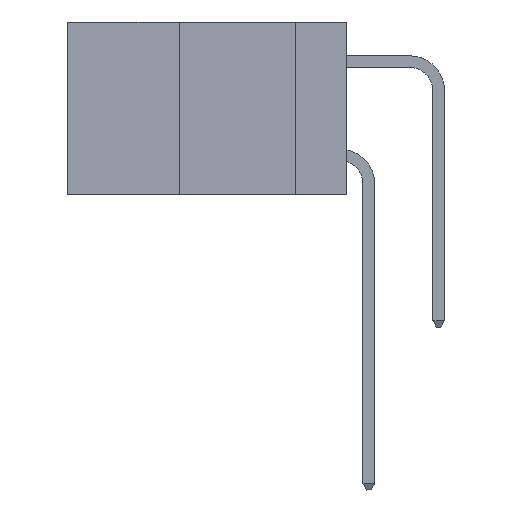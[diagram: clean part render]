
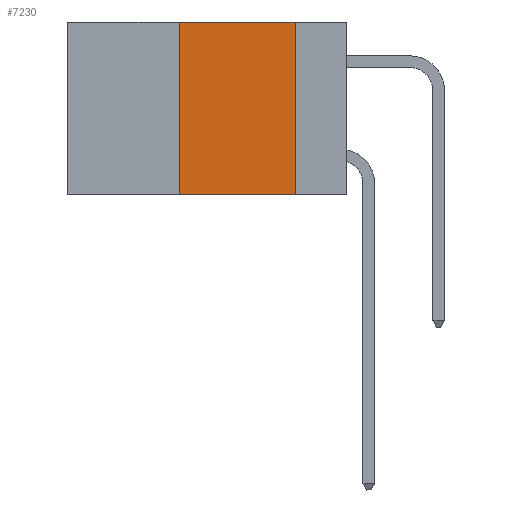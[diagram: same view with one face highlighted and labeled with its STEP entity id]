
A CAD part, left-side view. The second image highlights one B-rep face of the part: STEP entity #7230.
In plain terms, the highlighted planar face has unit normal (-1, 0, 0).
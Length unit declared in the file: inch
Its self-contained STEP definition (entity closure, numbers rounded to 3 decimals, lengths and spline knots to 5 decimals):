
#558 = VERTEX_POINT ( 'NONE', #15629 ) ;
#1822 = ORIENTED_EDGE ( 'NONE', *, *, #13832, .T. ) ;
#1832 = DIRECTION ( 'NONE',  ( 0., 0., -1. ) ) ;
#1865 = FACE_OUTER_BOUND ( 'NONE', #11019, .T. ) ;
#2364 = CARTESIAN_POINT ( 'NONE',  ( 0., 0.6, -0.37 ) ) ;
#2474 = DIRECTION ( 'NONE',  ( 0., -1., 0. ) ) ;
#3385 = VERTEX_POINT ( 'NONE', #8824 ) ;
#3894 = DIRECTION ( 'NONE',  ( 0., -1., 0. ) ) ;
#4068 = CARTESIAN_POINT ( 'NONE',  ( 0., 0.6, 0. ) ) ;
#4697 = VECTOR ( 'NONE', #3894, 39.37008 ) ;
#5134 = ORIENTED_EDGE ( 'NONE', *, *, #15643, .F. ) ;
#5179 = LINE ( 'NONE', #2364, #4697 ) ;
#6358 = CARTESIAN_POINT ( 'NONE',  ( 0., 0.11, 0. ) ) ;
#6613 = VERTEX_POINT ( 'NONE', #8448 ) ;
#6871 = VERTEX_POINT ( 'NONE', #9005 ) ;
#6977 = EDGE_CURVE ( 'NONE', #6871, #558, #10029, .T. ) ;
#6983 = PLANE ( 'NONE',  #18477 ) ;
#7230 = ADVANCED_FACE ( 'NONE', ( #1865 ), #6983, .F. ) ;
#7752 = VECTOR ( 'NONE', #2474, 39.37008 ) ;
#8200 = LINE ( 'NONE', #4068, #7752 ) ;
#8424 = DIRECTION ( 'NONE',  ( 0., 0., -1. ) ) ;
#8448 = CARTESIAN_POINT ( 'NONE',  ( 0., 0.36, -0.37 ) ) ;
#8824 = CARTESIAN_POINT ( 'NONE',  ( 0., 0.36, 0. ) ) ;
#9005 = CARTESIAN_POINT ( 'NONE',  ( 0., 0.11, 0. ) ) ;
#9834 = CARTESIAN_POINT ( 'NONE',  ( 0., 0.6, 0. ) ) ;
#10022 = CARTESIAN_POINT ( 'NONE',  ( 0., 0.36, 0. ) ) ;
#10029 = LINE ( 'NONE', #6358, #17221 ) ;
#11019 = EDGE_LOOP ( 'NONE', ( #17334, #18009, #5134, #1822 ) ) ;
#12749 = EDGE_CURVE ( 'NONE', #3385, #6871, #8200, .T. ) ;
#13832 = EDGE_CURVE ( 'NONE', #6613, #558, #5179, .T. ) ;
#13918 = VECTOR ( 'NONE', #16676, 39.37008 ) ;
#14335 = LINE ( 'NONE', #10022, #13918 ) ;
#15629 = CARTESIAN_POINT ( 'NONE',  ( 0., 0.11, -0.37 ) ) ;
#15643 = EDGE_CURVE ( 'NONE', #6613, #3385, #14335, .T. ) ;
#16617 = DIRECTION ( 'NONE',  ( 1., 0., 0. ) ) ;
#16676 = DIRECTION ( 'NONE',  ( 0., 0., 1. ) ) ;
#17221 = VECTOR ( 'NONE', #1832, 39.37008 ) ;
#17334 = ORIENTED_EDGE ( 'NONE', *, *, #6977, .F. ) ;
#18009 = ORIENTED_EDGE ( 'NONE', *, *, #12749, .F. ) ;
#18477 = AXIS2_PLACEMENT_3D ( 'NONE', #9834, #16617, #8424 ) ;
